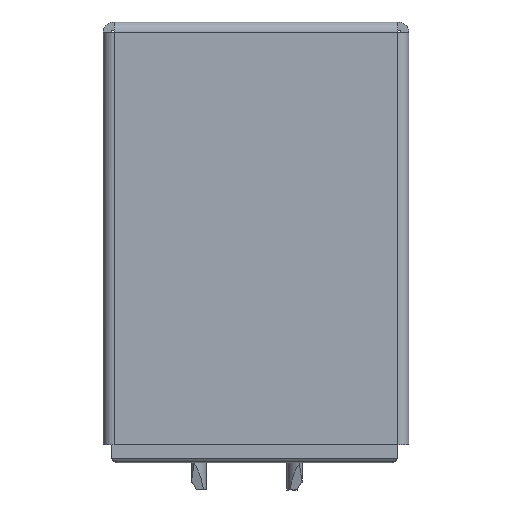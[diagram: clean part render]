
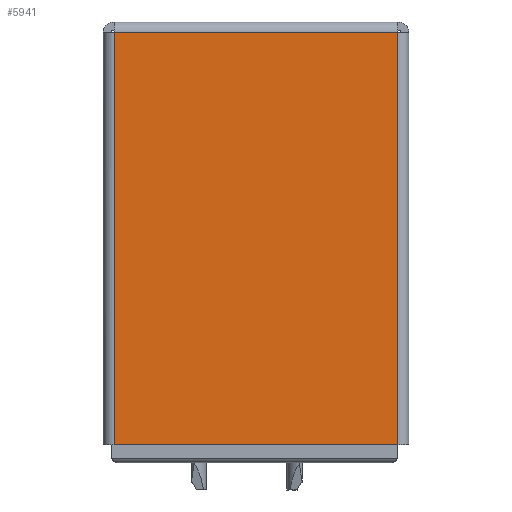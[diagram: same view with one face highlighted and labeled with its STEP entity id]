
A CAD part, left-side view. The second image highlights one B-rep face of the part: STEP entity #5941.
In plain terms, the highlighted face is planar.
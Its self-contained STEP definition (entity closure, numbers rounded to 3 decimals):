
#135 = VECTOR ( 'NONE', #8789, 1000. ) ;
#472 = ORIENTED_EDGE ( 'NONE', *, *, #5481, .F. ) ;
#539 = LINE ( 'NONE', #5539, #6548 ) ;
#610 = DIRECTION ( 'NONE',  ( 0., 0., 1. ) ) ;
#947 = LINE ( 'NONE', #9385, #2690 ) ;
#993 = VECTOR ( 'NONE', #8801, 1000. ) ;
#1029 = DIRECTION ( 'NONE',  ( 0., 0., -1. ) ) ;
#1295 = LINE ( 'NONE', #6055, #10341 ) ;
#1490 = CARTESIAN_POINT ( 'NONE',  ( 20.44, -0.24, -10.958 ) ) ;
#1578 = DIRECTION ( 'NONE',  ( 0., -1., 0. ) ) ;
#2140 = VERTEX_POINT ( 'NONE', #13911 ) ;
#2354 = FACE_OUTER_BOUND ( 'NONE', #2483, .T. ) ;
#2483 = EDGE_LOOP ( 'NONE', ( #15801, #472, #7889, #14761, #7030, #10268 ) ) ;
#2690 = VECTOR ( 'NONE', #610, 1000. ) ;
#3567 = PLANE ( 'NONE',  #5174 ) ;
#4031 = EDGE_CURVE ( 'NONE', #2140, #14743, #539, .T. ) ;
#4661 = VERTEX_POINT ( 'NONE', #12677 ) ;
#4909 = DIRECTION ( 'NONE',  ( 0., 0., 1. ) ) ;
#5174 = AXIS2_PLACEMENT_3D ( 'NONE', #1490, #1578, #12273 ) ;
#5455 = VERTEX_POINT ( 'NONE', #6291 ) ;
#5481 = EDGE_CURVE ( 'NONE', #5455, #4661, #1295, .T. ) ;
#5539 = CARTESIAN_POINT ( 'NONE',  ( 12.588, -0.24, -10.75 ) ) ;
#5941 = ADVANCED_FACE ( 'NONE', ( #2354 ), #3567, .T. ) ;
#6014 = CARTESIAN_POINT ( 'NONE',  ( 20.138, -0.24, -0.35 ) ) ;
#6055 = CARTESIAN_POINT ( 'NONE',  ( 5.038, -0.24, -5.55 ) ) ;
#6291 = CARTESIAN_POINT ( 'NONE',  ( 5.038, -0.24, -0.363 ) ) ;
#6548 = VECTOR ( 'NONE', #9299, 1000. ) ;
#6822 = VERTEX_POINT ( 'NONE', #11092 ) ;
#7030 = ORIENTED_EDGE ( 'NONE', *, *, #4031, .T. ) ;
#7488 = LINE ( 'NONE', #12501, #993 ) ;
#7889 = ORIENTED_EDGE ( 'NONE', *, *, #14170, .T. ) ;
#8176 = CARTESIAN_POINT ( 'NONE',  ( 20.138, -0.24, -10.75 ) ) ;
#8714 = LINE ( 'NONE', #14900, #135 ) ;
#8789 = DIRECTION ( 'NONE',  ( 0., 0., -1. ) ) ;
#8801 = DIRECTION ( 'NONE',  ( -1., 0., 0. ) ) ;
#8829 = EDGE_CURVE ( 'NONE', #13019, #4661, #7488, .T. ) ;
#9299 = DIRECTION ( 'NONE',  ( 1., 0., 0. ) ) ;
#9385 = CARTESIAN_POINT ( 'NONE',  ( 20.138, -0.24, -5.55 ) ) ;
#10268 = ORIENTED_EDGE ( 'NONE', *, *, #12763, .T. ) ;
#10341 = VECTOR ( 'NONE', #4909, 1000. ) ;
#11092 = CARTESIAN_POINT ( 'NONE',  ( 5.038, -0.24, -10.737 ) ) ;
#12273 = DIRECTION ( 'NONE',  ( 0., 0., 1. ) ) ;
#12501 = CARTESIAN_POINT ( 'NONE',  ( 12.538, -0.24, -0.35 ) ) ;
#12677 = CARTESIAN_POINT ( 'NONE',  ( 5.038, -0.24, -0.35 ) ) ;
#12763 = EDGE_CURVE ( 'NONE', #14743, #13019, #947, .T. ) ;
#13019 = VERTEX_POINT ( 'NONE', #6014 ) ;
#13911 = CARTESIAN_POINT ( 'NONE',  ( 5.038, -0.24, -10.75 ) ) ;
#14170 = EDGE_CURVE ( 'NONE', #5455, #6822, #8714, .T. ) ;
#14328 = VECTOR ( 'NONE', #1029, 1000. ) ;
#14739 = CARTESIAN_POINT ( 'NONE',  ( 5.038, -0.24, -5.55 ) ) ;
#14743 = VERTEX_POINT ( 'NONE', #8176 ) ;
#14761 = ORIENTED_EDGE ( 'NONE', *, *, #15984, .T. ) ;
#14900 = CARTESIAN_POINT ( 'NONE',  ( 5.038, -0.24, -5.55 ) ) ;
#15801 = ORIENTED_EDGE ( 'NONE', *, *, #8829, .T. ) ;
#15823 = LINE ( 'NONE', #14739, #14328 ) ;
#15984 = EDGE_CURVE ( 'NONE', #6822, #2140, #15823, .T. ) ;
